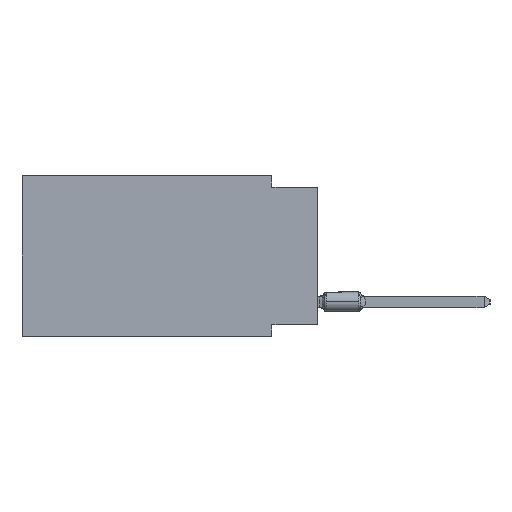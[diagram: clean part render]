
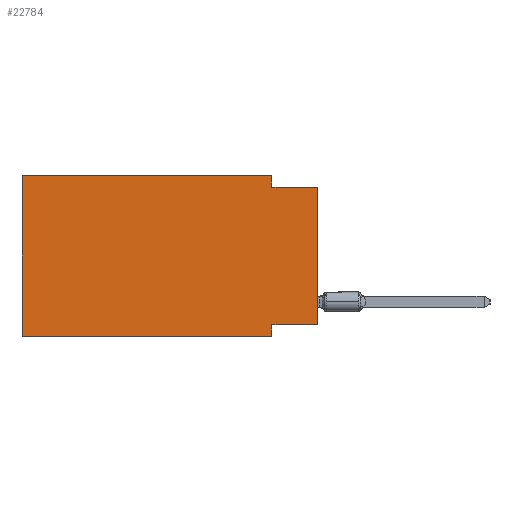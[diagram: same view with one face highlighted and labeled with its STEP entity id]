
A CAD part, left-side view. The second image highlights one B-rep face of the part: STEP entity #22784.
In plain terms, the highlighted planar face has unit normal (-1, 0, 0).
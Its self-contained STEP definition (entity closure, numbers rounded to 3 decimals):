
#4190 = VECTOR ( 'NONE', #33613, 1000. ) ;
#4563 = DIRECTION ( 'NONE',  ( 0., -1., 0. ) ) ;
#5207 = CARTESIAN_POINT ( 'NONE',  ( 0., 0., 0. ) ) ;
#5374 = DIRECTION ( 'NONE',  ( 0., -1., 0. ) ) ;
#5515 = EDGE_CURVE ( 'NONE', #8689, #34221, #13729, .T. ) ;
#5628 = VERTEX_POINT ( 'NONE', #14081 ) ;
#6739 = CARTESIAN_POINT ( 'NONE',  ( 0., 2.54, -8.89 ) ) ;
#7820 = ORIENTED_EDGE ( 'NONE', *, *, #14905, .F. ) ;
#8559 = FACE_OUTER_BOUND ( 'NONE', #26412, .T. ) ;
#8689 = VERTEX_POINT ( 'NONE', #28802 ) ;
#8764 = ORIENTED_EDGE ( 'NONE', *, *, #25198, .F. ) ;
#9640 = LINE ( 'NONE', #25631, #4190 ) ;
#10071 = EDGE_CURVE ( 'NONE', #8689, #28073, #26606, .T. ) ;
#10175 = CARTESIAN_POINT ( 'NONE',  ( 0., 2.54, 0. ) ) ;
#10714 = DIRECTION ( 'NONE',  ( 0., 0., 1. ) ) ;
#10890 = CARTESIAN_POINT ( 'NONE',  ( 0., 16.383, -8.89 ) ) ;
#11682 = ORIENTED_EDGE ( 'NONE', *, *, #12089, .F. ) ;
#12089 = EDGE_CURVE ( 'NONE', #28073, #18676, #12207, .T. ) ;
#12207 = LINE ( 'NONE', #23052, #15429 ) ;
#12375 = ORIENTED_EDGE ( 'NONE', *, *, #31651, .T. ) ;
#13470 = ORIENTED_EDGE ( 'NONE', *, *, #10071, .F. ) ;
#13717 = PLANE ( 'NONE',  #14293 ) ;
#13729 = LINE ( 'NONE', #10890, #34429 ) ;
#14081 = CARTESIAN_POINT ( 'NONE',  ( 0., 0., -0.635 ) ) ;
#14293 = AXIS2_PLACEMENT_3D ( 'NONE', #30233, #24549, #32724 ) ;
#14526 = DIRECTION ( 'NONE',  ( 0., 0., -1. ) ) ;
#14579 = DIRECTION ( 'NONE',  ( 0., 1., 0. ) ) ;
#14905 = EDGE_CURVE ( 'NONE', #24448, #5628, #34367, .T. ) ;
#15032 = DIRECTION ( 'NONE',  ( 0., -1., 0. ) ) ;
#15429 = VECTOR ( 'NONE', #4563, 1000. ) ;
#17234 = CARTESIAN_POINT ( 'NONE',  ( 0., 0., -8.255 ) ) ;
#17862 = CARTESIAN_POINT ( 'NONE',  ( 0., 0., -0.635 ) ) ;
#18676 = VERTEX_POINT ( 'NONE', #10175 ) ;
#18701 = VECTOR ( 'NONE', #27778, 1000. ) ;
#19477 = ORIENTED_EDGE ( 'NONE', *, *, #30833, .F. ) ;
#21075 = CARTESIAN_POINT ( 'NONE',  ( 0., 0., -8.255 ) ) ;
#21104 = ORIENTED_EDGE ( 'NONE', *, *, #5515, .T. ) ;
#22784 = ADVANCED_FACE ( 'NONE', ( #8559 ), #13717, .F. ) ;
#22915 = CARTESIAN_POINT ( 'NONE',  ( 0., 2.54, -0.635 ) ) ;
#23052 = CARTESIAN_POINT ( 'NONE',  ( 0., 16.383, 0. ) ) ;
#23460 = VECTOR ( 'NONE', #14579, 1000. ) ;
#24219 = LINE ( 'NONE', #5207, #33284 ) ;
#24448 = VERTEX_POINT ( 'NONE', #22915 ) ;
#24549 = DIRECTION ( 'NONE',  ( 1., 0., 0. ) ) ;
#25182 = LINE ( 'NONE', #33527, #30566 ) ;
#25198 = EDGE_CURVE ( 'NONE', #28053, #34221, #9640, .T. ) ;
#25631 = CARTESIAN_POINT ( 'NONE',  ( 0., 2.54, -8.89 ) ) ;
#26056 = EDGE_CURVE ( 'NONE', #26633, #28053, #30742, .T. ) ;
#26412 = EDGE_LOOP ( 'NONE', ( #12375, #7820, #19477, #11682, #13470, #21104, #8764, #31727 ) ) ;
#26606 = LINE ( 'NONE', #34756, #18701 ) ;
#26633 = VERTEX_POINT ( 'NONE', #21075 ) ;
#27778 = DIRECTION ( 'NONE',  ( 0., 0., 1. ) ) ;
#27822 = CARTESIAN_POINT ( 'NONE',  ( 0., 16.383, 0. ) ) ;
#28053 = VERTEX_POINT ( 'NONE', #30133 ) ;
#28073 = VERTEX_POINT ( 'NONE', #27822 ) ;
#28802 = CARTESIAN_POINT ( 'NONE',  ( 0., 16.383, -8.89 ) ) ;
#30133 = CARTESIAN_POINT ( 'NONE',  ( 0., 2.54, -8.255 ) ) ;
#30233 = CARTESIAN_POINT ( 'NONE',  ( 0., 16.383, 0. ) ) ;
#30566 = VECTOR ( 'NONE', #14526, 1000. ) ;
#30742 = LINE ( 'NONE', #17234, #23460 ) ;
#30833 = EDGE_CURVE ( 'NONE', #18676, #24448, #25182, .T. ) ;
#31651 = EDGE_CURVE ( 'NONE', #26633, #5628, #24219, .T. ) ;
#31727 = ORIENTED_EDGE ( 'NONE', *, *, #26056, .F. ) ;
#32724 = DIRECTION ( 'NONE',  ( 0., 0., -1. ) ) ;
#33284 = VECTOR ( 'NONE', #10714, 1000. ) ;
#33527 = CARTESIAN_POINT ( 'NONE',  ( 0., 2.54, 0. ) ) ;
#33613 = DIRECTION ( 'NONE',  ( 0., 0., -1. ) ) ;
#34221 = VERTEX_POINT ( 'NONE', #6739 ) ;
#34367 = LINE ( 'NONE', #17862, #34818 ) ;
#34429 = VECTOR ( 'NONE', #5374, 1000. ) ;
#34756 = CARTESIAN_POINT ( 'NONE',  ( 0., 16.383, 0. ) ) ;
#34818 = VECTOR ( 'NONE', #15032, 1000. ) ;
